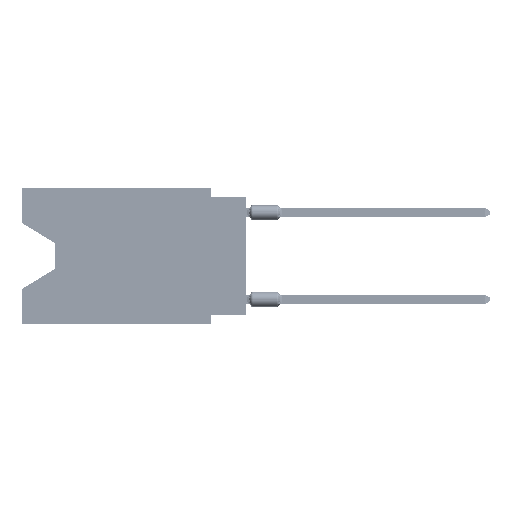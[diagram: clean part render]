
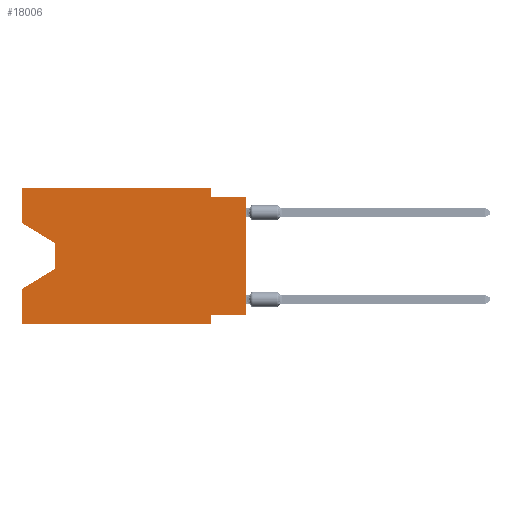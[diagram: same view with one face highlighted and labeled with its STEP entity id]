
A CAD part, left-side view. The second image highlights one B-rep face of the part: STEP entity #18006.
In plain terms, the highlighted planar face has unit normal (-1, 0, 0).
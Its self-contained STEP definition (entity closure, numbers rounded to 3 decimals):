
#1084 = DIRECTION ( 'NONE',  ( 0., -1., 0. ) ) ;
#1722 = LINE ( 'NONE', #42870, #58037 ) ;
#1755 = LINE ( 'NONE', #15059, #65750 ) ;
#2634 = VECTOR ( 'NONE', #17825, 1000. ) ;
#2660 = CARTESIAN_POINT ( 'NONE',  ( 0., 13.97, -5.893 ) ) ;
#3437 = VECTOR ( 'NONE', #41951, 1000. ) ;
#3471 = DIRECTION ( 'NONE',  ( 0., 0., -1. ) ) ;
#3831 = CARTESIAN_POINT ( 'NONE',  ( 0., 16.383, -2.546 ) ) ;
#4764 = VERTEX_POINT ( 'NONE', #6368 ) ;
#4856 = CARTESIAN_POINT ( 'NONE',  ( 0., 16.383, 0. ) ) ;
#6368 = CARTESIAN_POINT ( 'NONE',  ( 0., 2.54, -0.635 ) ) ;
#8732 = VERTEX_POINT ( 'NONE', #58153 ) ;
#9636 = VECTOR ( 'NONE', #49714, 1000. ) ;
#10087 = ORIENTED_EDGE ( 'NONE', *, *, #27087, .F. ) ;
#11614 = DIRECTION ( 'NONE',  ( 0., -1., 0. ) ) ;
#11956 = CARTESIAN_POINT ( 'NONE',  ( 0., 13.97, -4.013 ) ) ;
#11980 = DIRECTION ( 'NONE',  ( 0., 1., 0. ) ) ;
#12490 = ORIENTED_EDGE ( 'NONE', *, *, #22065, .F. ) ;
#13595 = ORIENTED_EDGE ( 'NONE', *, *, #68059, .T. ) ;
#14397 = AXIS2_PLACEMENT_3D ( 'NONE', #4856, #52697, #76590 ) ;
#15059 = CARTESIAN_POINT ( 'NONE',  ( 0., 2.54, -9.906 ) ) ;
#15388 = EDGE_CURVE ( 'NONE', #72667, #40740, #76172, .T. ) ;
#16911 = ORIENTED_EDGE ( 'NONE', *, *, #15388, .T. ) ;
#17825 = DIRECTION ( 'NONE',  ( 0., 0., 1. ) ) ;
#18006 = ADVANCED_FACE ( 'NONE', ( #53098 ), #33478, .F. ) ;
#20087 = VERTEX_POINT ( 'NONE', #49062 ) ;
#20953 = DIRECTION ( 'NONE',  ( 0., 0., -1. ) ) ;
#21822 = VERTEX_POINT ( 'NONE', #3831 ) ;
#22017 = ORIENTED_EDGE ( 'NONE', *, *, #33825, .F. ) ;
#22065 = EDGE_CURVE ( 'NONE', #4764, #43150, #37523, .T. ) ;
#24599 = ORIENTED_EDGE ( 'NONE', *, *, #35659, .T. ) ;
#25352 = VECTOR ( 'NONE', #20953, 1000. ) ;
#26495 = VECTOR ( 'NONE', #11980, 1000. ) ;
#27087 = EDGE_CURVE ( 'NONE', #71776, #52919, #47598, .T. ) ;
#27354 = EDGE_CURVE ( 'NONE', #48366, #20087, #40468, .T. ) ;
#29494 = DIRECTION ( 'NONE',  ( 0., -1., 0. ) ) ;
#31181 = VERTEX_POINT ( 'NONE', #65253 ) ;
#31672 = VECTOR ( 'NONE', #3471, 1000. ) ;
#33478 = PLANE ( 'NONE',  #14397 ) ;
#33825 = EDGE_CURVE ( 'NONE', #31181, #61815, #1755, .T. ) ;
#33917 = VECTOR ( 'NONE', #34718, 1000. ) ;
#34718 = DIRECTION ( 'NONE',  ( 0., 0., 1. ) ) ;
#35659 = EDGE_CURVE ( 'NONE', #40740, #52919, #37943, .T. ) ;
#36607 = VECTOR ( 'NONE', #29494, 1000. ) ;
#36906 = EDGE_CURVE ( 'NONE', #21822, #72667, #76451, .T. ) ;
#37031 = LINE ( 'NONE', #60543, #26495 ) ;
#37523 = LINE ( 'NONE', #61431, #77358 ) ;
#37943 = LINE ( 'NONE', #2660, #9636 ) ;
#40468 = LINE ( 'NONE', #75724, #36607 ) ;
#40640 = EDGE_CURVE ( 'NONE', #71776, #61815, #47284, .T. ) ;
#40740 = VERTEX_POINT ( 'NONE', #56436 ) ;
#41786 = CARTESIAN_POINT ( 'NONE',  ( 0., 16.383, 0. ) ) ;
#41951 = DIRECTION ( 'NONE',  ( 0., -0.855, -0.519 ) ) ;
#42870 = CARTESIAN_POINT ( 'NONE',  ( 0., 0., 0. ) ) ;
#43150 = VERTEX_POINT ( 'NONE', #60865 ) ;
#43627 = CARTESIAN_POINT ( 'NONE',  ( 0., 2.54, -9.906 ) ) ;
#43803 = EDGE_CURVE ( 'NONE', #20087, #4764, #63081, .T. ) ;
#47284 = LINE ( 'NONE', #71189, #53735 ) ;
#47598 = LINE ( 'NONE', #71506, #2634 ) ;
#48366 = VERTEX_POINT ( 'NONE', #41786 ) ;
#49062 = CARTESIAN_POINT ( 'NONE',  ( 0., 2.54, 0. ) ) ;
#49714 = DIRECTION ( 'NONE',  ( 0., 0.855, -0.519 ) ) ;
#52697 = DIRECTION ( 'NONE',  ( 1., 0., 0. ) ) ;
#52739 = LINE ( 'NONE', #64879, #33917 ) ;
#52919 = VERTEX_POINT ( 'NONE', #68025 ) ;
#53079 = EDGE_CURVE ( 'NONE', #21822, #48366, #52739, .T. ) ;
#53098 = FACE_OUTER_BOUND ( 'NONE', #60310, .T. ) ;
#53724 = CARTESIAN_POINT ( 'NONE',  ( 0., 16.383, -2.546 ) ) ;
#53735 = VECTOR ( 'NONE', #11614, 1000. ) ;
#54426 = EDGE_CURVE ( 'NONE', #8732, #31181, #37031, .T. ) ;
#54948 = CARTESIAN_POINT ( 'NONE',  ( 0., 16.383, -9.906 ) ) ;
#55419 = DIRECTION ( 'NONE',  ( 0., 0., 1. ) ) ;
#56436 = CARTESIAN_POINT ( 'NONE',  ( 0., 13.97, -5.893 ) ) ;
#57789 = ORIENTED_EDGE ( 'NONE', *, *, #27354, .F. ) ;
#58037 = VECTOR ( 'NONE', #55419, 1000. ) ;
#58153 = CARTESIAN_POINT ( 'NONE',  ( 0., 0., -9.271 ) ) ;
#58760 = CARTESIAN_POINT ( 'NONE',  ( 0., 2.54, 0. ) ) ;
#60310 = EDGE_LOOP ( 'NONE', ( #64356, #16911, #24599, #10087, #76098, #22017, #67058, #13595, #12490, #73692, #57789, #71197 ) ) ;
#60543 = CARTESIAN_POINT ( 'NONE',  ( 0., 0., -9.271 ) ) ;
#60865 = CARTESIAN_POINT ( 'NONE',  ( 0., 0., -0.635 ) ) ;
#61431 = CARTESIAN_POINT ( 'NONE',  ( 0., 0., -0.635 ) ) ;
#61815 = VERTEX_POINT ( 'NONE', #43627 ) ;
#63081 = LINE ( 'NONE', #58760, #31672 ) ;
#64356 = ORIENTED_EDGE ( 'NONE', *, *, #36906, .T. ) ;
#64879 = CARTESIAN_POINT ( 'NONE',  ( 0., 16.383, 0. ) ) ;
#65253 = CARTESIAN_POINT ( 'NONE',  ( 0., 2.54, -9.271 ) ) ;
#65750 = VECTOR ( 'NONE', #67957, 1000. ) ;
#67058 = ORIENTED_EDGE ( 'NONE', *, *, #54426, .F. ) ;
#67957 = DIRECTION ( 'NONE',  ( 0., 0., -1. ) ) ;
#68025 = CARTESIAN_POINT ( 'NONE',  ( 0., 16.383, -7.36 ) ) ;
#68059 = EDGE_CURVE ( 'NONE', #8732, #43150, #1722, .T. ) ;
#69887 = CARTESIAN_POINT ( 'NONE',  ( 0., 13.97, -4.013 ) ) ;
#71189 = CARTESIAN_POINT ( 'NONE',  ( 0., 16.383, -9.906 ) ) ;
#71197 = ORIENTED_EDGE ( 'NONE', *, *, #53079, .F. ) ;
#71506 = CARTESIAN_POINT ( 'NONE',  ( 0., 16.383, 0. ) ) ;
#71776 = VERTEX_POINT ( 'NONE', #54948 ) ;
#72667 = VERTEX_POINT ( 'NONE', #11956 ) ;
#73692 = ORIENTED_EDGE ( 'NONE', *, *, #43803, .F. ) ;
#75724 = CARTESIAN_POINT ( 'NONE',  ( 0., 16.383, 0. ) ) ;
#76098 = ORIENTED_EDGE ( 'NONE', *, *, #40640, .T. ) ;
#76172 = LINE ( 'NONE', #69887, #25352 ) ;
#76451 = LINE ( 'NONE', #53724, #3437 ) ;
#76590 = DIRECTION ( 'NONE',  ( 0., 0., -1. ) ) ;
#77358 = VECTOR ( 'NONE', #1084, 1000. ) ;
